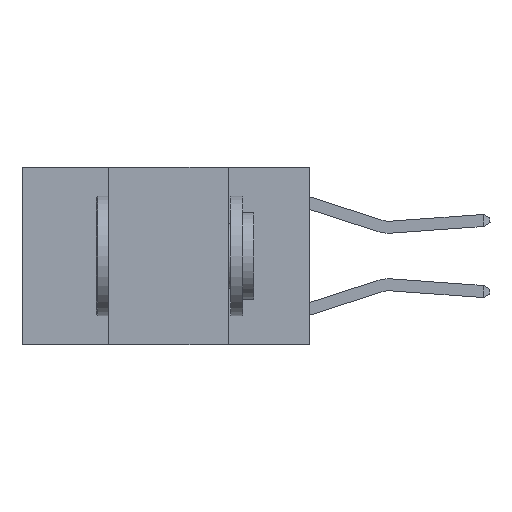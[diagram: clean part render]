
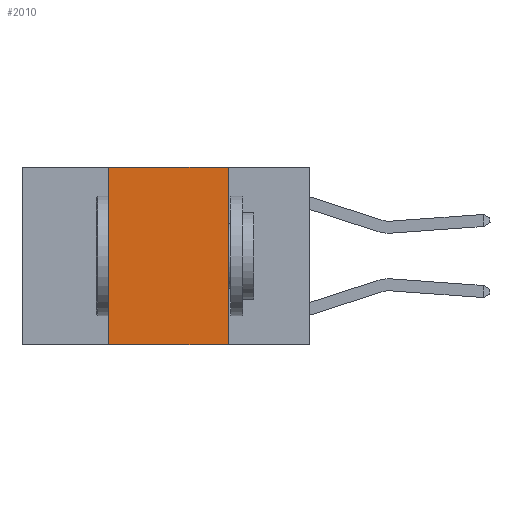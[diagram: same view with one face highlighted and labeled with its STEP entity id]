
A CAD part, left-side view. The second image highlights one B-rep face of the part: STEP entity #2010.
In plain terms, the highlighted planar face has unit normal (-1, 0, 0).
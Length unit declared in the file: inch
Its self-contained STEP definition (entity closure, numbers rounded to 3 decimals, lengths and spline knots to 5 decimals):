
#836 = CARTESIAN_POINT ( 'NONE',  ( 0., 0.17, 0. ) ) ;
#907 = CARTESIAN_POINT ( 'NONE',  ( 0., 0.42, 0. ) ) ;
#928 = AXIS2_PLACEMENT_3D ( 'NONE', #9478, #9055, #8918 ) ;
#1311 = LINE ( 'NONE', #7718, #11084 ) ;
#1633 = VERTEX_POINT ( 'NONE', #10892 ) ;
#1723 = LINE ( 'NONE', #6153, #11374 ) ;
#1930 = VERTEX_POINT ( 'NONE', #3276 ) ;
#2010 = ADVANCED_FACE ( 'NONE', ( #5306 ), #9331, .F. ) ;
#2046 = EDGE_CURVE ( 'NONE', #8055, #8778, #1723, .T. ) ;
#3276 = CARTESIAN_POINT ( 'NONE',  ( 0., 0.42, -0.37 ) ) ;
#3448 = ORIENTED_EDGE ( 'NONE', *, *, #7925, .F. ) ;
#3469 = ORIENTED_EDGE ( 'NONE', *, *, #2046, .F. ) ;
#3568 = ORIENTED_EDGE ( 'NONE', *, *, #7945, .F. ) ;
#3606 = ORIENTED_EDGE ( 'NONE', *, *, #8389, .T. ) ;
#3730 = VECTOR ( 'NONE', #4875, 39.37008 ) ;
#4833 = DIRECTION ( 'NONE',  ( 0., 0., -1. ) ) ;
#4875 = DIRECTION ( 'NONE',  ( 0., 0., 1. ) ) ;
#5237 = LINE ( 'NONE', #10832, #12071 ) ;
#5306 = FACE_OUTER_BOUND ( 'NONE', #7199, .T. ) ;
#5992 = DIRECTION ( 'NONE',  ( 0., -1., 0. ) ) ;
#6153 = CARTESIAN_POINT ( 'NONE',  ( 0., 0.6, 0. ) ) ;
#6326 = LINE ( 'NONE', #6802, #3730 ) ;
#6365 = DIRECTION ( 'NONE',  ( 0., -1., 0. ) ) ;
#6802 = CARTESIAN_POINT ( 'NONE',  ( 0., 0.42, 0. ) ) ;
#7199 = EDGE_LOOP ( 'NONE', ( #3448, #3469, #3568, #3606 ) ) ;
#7718 = CARTESIAN_POINT ( 'NONE',  ( 0., 0.17, 0. ) ) ;
#7925 = EDGE_CURVE ( 'NONE', #8778, #1633, #1311, .T. ) ;
#7945 = EDGE_CURVE ( 'NONE', #1930, #8055, #6326, .T. ) ;
#8055 = VERTEX_POINT ( 'NONE', #907 ) ;
#8389 = EDGE_CURVE ( 'NONE', #1930, #1633, #5237, .T. ) ;
#8778 = VERTEX_POINT ( 'NONE', #836 ) ;
#8918 = DIRECTION ( 'NONE',  ( 0., 0., -1. ) ) ;
#9055 = DIRECTION ( 'NONE',  ( 1., 0., 0. ) ) ;
#9331 = PLANE ( 'NONE',  #928 ) ;
#9478 = CARTESIAN_POINT ( 'NONE',  ( 0., 0.6, 0. ) ) ;
#10832 = CARTESIAN_POINT ( 'NONE',  ( 0., 0.6, -0.37 ) ) ;
#10892 = CARTESIAN_POINT ( 'NONE',  ( 0., 0.17, -0.37 ) ) ;
#11084 = VECTOR ( 'NONE', #4833, 39.37008 ) ;
#11374 = VECTOR ( 'NONE', #5992, 39.37008 ) ;
#12071 = VECTOR ( 'NONE', #6365, 39.37008 ) ;
